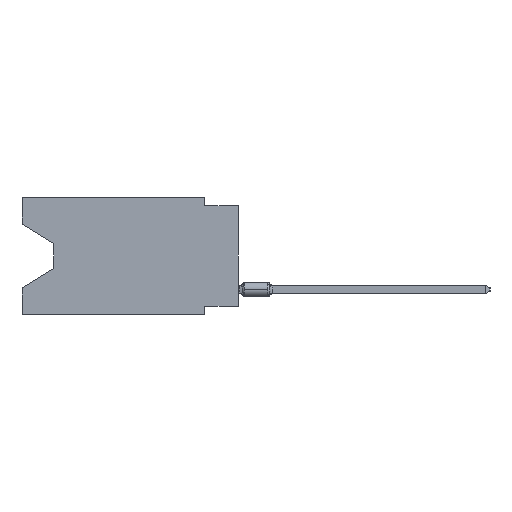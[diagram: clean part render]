
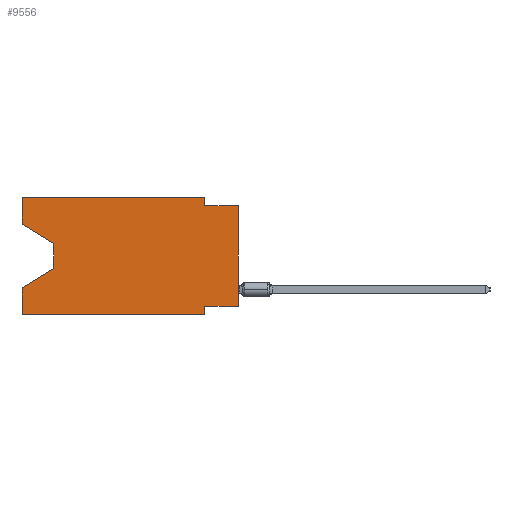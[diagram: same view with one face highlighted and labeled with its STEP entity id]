
A CAD part, left-side view. The second image highlights one B-rep face of the part: STEP entity #9556.
In plain terms, the highlighted planar face has unit normal (-1, 0, 0).
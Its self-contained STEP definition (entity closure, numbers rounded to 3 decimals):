
#1408 = ORIENTED_EDGE ( 'NONE', *, *, #36994, .T. ) ;
#1923 = EDGE_CURVE ( 'NONE', #4631, #11957, #4635, .T. ) ;
#2200 = VECTOR ( 'NONE', #26123, 1000. ) ;
#2773 = VECTOR ( 'NONE', #13332, 1000. ) ;
#2783 = CARTESIAN_POINT ( 'NONE',  ( 0., 13.97, -3.505 ) ) ;
#2807 = ORIENTED_EDGE ( 'NONE', *, *, #7227, .T. ) ;
#3785 = VERTEX_POINT ( 'NONE', #5298 ) ;
#4523 = ORIENTED_EDGE ( 'NONE', *, *, #22499, .T. ) ;
#4631 = VERTEX_POINT ( 'NONE', #43890 ) ;
#4635 = LINE ( 'NONE', #29087, #8999 ) ;
#5161 = DIRECTION ( 'NONE',  ( 0., 0., 1. ) ) ;
#5298 = CARTESIAN_POINT ( 'NONE',  ( 0., 2.54, -8.89 ) ) ;
#6008 = CARTESIAN_POINT ( 'NONE',  ( 0., 2.54, 0. ) ) ;
#6028 = LINE ( 'NONE', #40758, #2773 ) ;
#7040 = FACE_OUTER_BOUND ( 'NONE', #23511, .T. ) ;
#7227 = EDGE_CURVE ( 'NONE', #12564, #10020, #42089, .T. ) ;
#7824 = CARTESIAN_POINT ( 'NONE',  ( 0., 16.383, 0. ) ) ;
#8028 = ORIENTED_EDGE ( 'NONE', *, *, #27660, .F. ) ;
#8605 = DIRECTION ( 'NONE',  ( 0., 0., -1. ) ) ;
#8821 = VECTOR ( 'NONE', #44351, 1000. ) ;
#8999 = VECTOR ( 'NONE', #35489, 1000. ) ;
#9542 = LINE ( 'NONE', #36276, #38351 ) ;
#9556 = ADVANCED_FACE ( 'NONE', ( #7040 ), #28505, .F. ) ;
#10020 = VERTEX_POINT ( 'NONE', #25011 ) ;
#11555 = ORIENTED_EDGE ( 'NONE', *, *, #15961, .F. ) ;
#11813 = VECTOR ( 'NONE', #16167, 1000. ) ;
#11957 = VERTEX_POINT ( 'NONE', #29975 ) ;
#12564 = VERTEX_POINT ( 'NONE', #2783 ) ;
#12586 = CARTESIAN_POINT ( 'NONE',  ( 0., 16.383, -8.89 ) ) ;
#13332 = DIRECTION ( 'NONE',  ( 0., 0., 1. ) ) ;
#13771 = DIRECTION ( 'NONE',  ( 0., 0., -1. ) ) ;
#14169 = VECTOR ( 'NONE', #20214, 1000. ) ;
#14309 = VERTEX_POINT ( 'NONE', #7824 ) ;
#14963 = LINE ( 'NONE', #32757, #2200 ) ;
#15237 = CARTESIAN_POINT ( 'NONE',  ( 0., 16.383, 0. ) ) ;
#15928 = LINE ( 'NONE', #22976, #19968 ) ;
#15961 = EDGE_CURVE ( 'NONE', #11957, #3785, #15928, .T. ) ;
#16167 = DIRECTION ( 'NONE',  ( 0., 0.855, -0.519 ) ) ;
#16498 = DIRECTION ( 'NONE',  ( 0., -0.855, -0.519 ) ) ;
#16930 = LINE ( 'NONE', #22863, #26566 ) ;
#17111 = DIRECTION ( 'NONE',  ( 0., 0., -1. ) ) ;
#17191 = LINE ( 'NONE', #6008, #39882 ) ;
#17245 = CARTESIAN_POINT ( 'NONE',  ( 0., 16.383, -2.038 ) ) ;
#18336 = CARTESIAN_POINT ( 'NONE',  ( 0., 13.97, -3.505 ) ) ;
#19532 = CARTESIAN_POINT ( 'NONE',  ( 0., 2.54, 0. ) ) ;
#19968 = VECTOR ( 'NONE', #8605, 1000. ) ;
#20047 = LINE ( 'NONE', #40373, #11813 ) ;
#20214 = DIRECTION ( 'NONE',  ( 0., 0., 1. ) ) ;
#20972 = DIRECTION ( 'NONE',  ( 1., 0., 0. ) ) ;
#22499 = EDGE_CURVE ( 'NONE', #4631, #36060, #6028, .T. ) ;
#22863 = CARTESIAN_POINT ( 'NONE',  ( 0., 16.383, -2.038 ) ) ;
#22976 = CARTESIAN_POINT ( 'NONE',  ( 0., 2.54, -8.89 ) ) ;
#23511 = EDGE_LOOP ( 'NONE', ( #36806, #2807, #23625, #39855, #1408, #11555, #25275, #4523, #8028, #27236, #31696, #33545 ) ) ;
#23625 = ORIENTED_EDGE ( 'NONE', *, *, #31503, .T. ) ;
#24831 = CARTESIAN_POINT ( 'NONE',  ( 0., 16.383, 0. ) ) ;
#25011 = CARTESIAN_POINT ( 'NONE',  ( 0., 13.97, -5.385 ) ) ;
#25275 = ORIENTED_EDGE ( 'NONE', *, *, #1923, .F. ) ;
#26071 = VERTEX_POINT ( 'NONE', #19532 ) ;
#26123 = DIRECTION ( 'NONE',  ( 0., -1., 0. ) ) ;
#26566 = VECTOR ( 'NONE', #16498, 1000. ) ;
#27236 = ORIENTED_EDGE ( 'NONE', *, *, #37902, .F. ) ;
#27660 = EDGE_CURVE ( 'NONE', #33298, #36060, #14963, .T. ) ;
#28505 = PLANE ( 'NONE',  #42091 ) ;
#29087 = CARTESIAN_POINT ( 'NONE',  ( 0., 0., -8.255 ) ) ;
#29586 = CARTESIAN_POINT ( 'NONE',  ( 0., 0., -0.635 ) ) ;
#29975 = CARTESIAN_POINT ( 'NONE',  ( 0., 2.54, -8.255 ) ) ;
#30565 = DIRECTION ( 'NONE',  ( 0., -1., 0. ) ) ;
#30713 = LINE ( 'NONE', #33924, #14169 ) ;
#30737 = EDGE_CURVE ( 'NONE', #14309, #26071, #41156, .T. ) ;
#31503 = EDGE_CURVE ( 'NONE', #10020, #39365, #20047, .T. ) ;
#31696 = ORIENTED_EDGE ( 'NONE', *, *, #30737, .F. ) ;
#32267 = DIRECTION ( 'NONE',  ( 0., 0., -1. ) ) ;
#32470 = CARTESIAN_POINT ( 'NONE',  ( 0., 16.383, -6.852 ) ) ;
#32587 = LINE ( 'NONE', #15237, #37419 ) ;
#32757 = CARTESIAN_POINT ( 'NONE',  ( 0., 0., -0.635 ) ) ;
#33273 = VECTOR ( 'NONE', #32267, 1000. ) ;
#33298 = VERTEX_POINT ( 'NONE', #43663 ) ;
#33388 = EDGE_CURVE ( 'NONE', #37578, #12564, #16930, .T. ) ;
#33545 = ORIENTED_EDGE ( 'NONE', *, *, #35213, .F. ) ;
#33924 = CARTESIAN_POINT ( 'NONE',  ( 0., 16.383, 0. ) ) ;
#35213 = EDGE_CURVE ( 'NONE', #37578, #14309, #30713, .T. ) ;
#35489 = DIRECTION ( 'NONE',  ( 0., 1., 0. ) ) ;
#36060 = VERTEX_POINT ( 'NONE', #29586 ) ;
#36276 = CARTESIAN_POINT ( 'NONE',  ( 0., 16.383, -8.89 ) ) ;
#36806 = ORIENTED_EDGE ( 'NONE', *, *, #33388, .T. ) ;
#36994 = EDGE_CURVE ( 'NONE', #42295, #3785, #9542, .T. ) ;
#37419 = VECTOR ( 'NONE', #5161, 1000. ) ;
#37578 = VERTEX_POINT ( 'NONE', #17245 ) ;
#37902 = EDGE_CURVE ( 'NONE', #26071, #33298, #17191, .T. ) ;
#38351 = VECTOR ( 'NONE', #30565, 1000. ) ;
#39365 = VERTEX_POINT ( 'NONE', #32470 ) ;
#39855 = ORIENTED_EDGE ( 'NONE', *, *, #43481, .F. ) ;
#39882 = VECTOR ( 'NONE', #13771, 1000. ) ;
#40373 = CARTESIAN_POINT ( 'NONE',  ( 0., 13.97, -5.385 ) ) ;
#40758 = CARTESIAN_POINT ( 'NONE',  ( 0., 0., 0. ) ) ;
#41156 = LINE ( 'NONE', #44121, #8821 ) ;
#42089 = LINE ( 'NONE', #18336, #33273 ) ;
#42091 = AXIS2_PLACEMENT_3D ( 'NONE', #24831, #20972, #17111 ) ;
#42295 = VERTEX_POINT ( 'NONE', #12586 ) ;
#43481 = EDGE_CURVE ( 'NONE', #42295, #39365, #32587, .T. ) ;
#43663 = CARTESIAN_POINT ( 'NONE',  ( 0., 2.54, -0.635 ) ) ;
#43890 = CARTESIAN_POINT ( 'NONE',  ( 0., 0., -8.255 ) ) ;
#44121 = CARTESIAN_POINT ( 'NONE',  ( 0., 16.383, 0. ) ) ;
#44351 = DIRECTION ( 'NONE',  ( 0., -1., 0. ) ) ;
